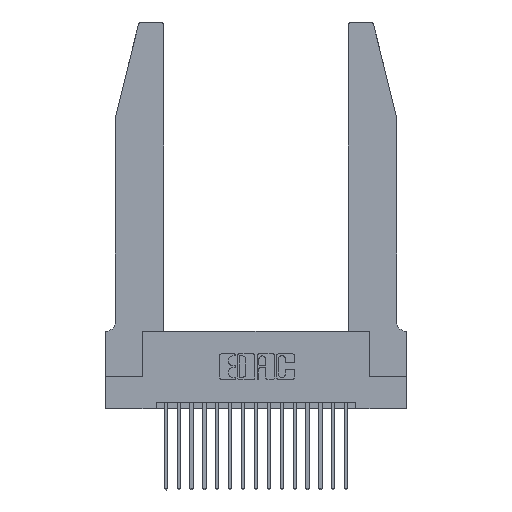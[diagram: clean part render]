
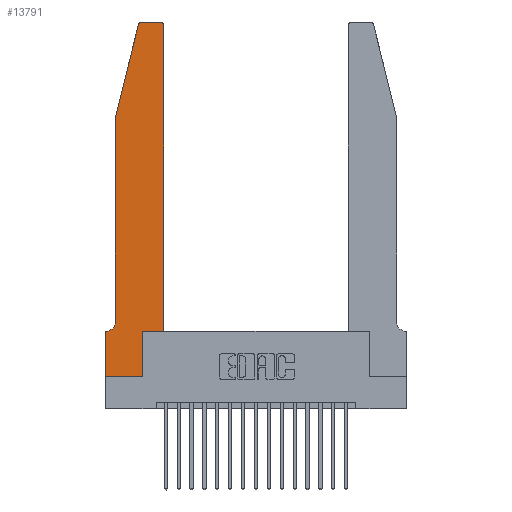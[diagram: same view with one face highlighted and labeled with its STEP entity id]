
A CAD part, top view. The second image highlights one B-rep face of the part: STEP entity #13791.
In plain terms, the highlighted planar face has unit normal (0, 0, 1).
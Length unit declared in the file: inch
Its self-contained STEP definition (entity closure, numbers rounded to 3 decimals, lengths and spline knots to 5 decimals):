
#321 = VECTOR ( 'NONE', #2564, 39.37008 ) ;
#482 = DIRECTION ( 'NONE',  ( 0., 0., 1. ) ) ;
#614 = DIRECTION ( 'NONE',  ( 1., 0., 0. ) ) ;
#712 = LINE ( 'NONE', #5059, #16830 ) ;
#840 = EDGE_CURVE ( 'NONE', #8991, #19075, #1540, .T. ) ;
#1194 = LINE ( 'NONE', #5356, #11461 ) ;
#1308 = DIRECTION ( 'NONE',  ( -0.239, -0.971, 0. ) ) ;
#1516 = VERTEX_POINT ( 'NONE', #19237 ) ;
#1540 = LINE ( 'NONE', #11918, #321 ) ;
#1639 = EDGE_CURVE ( 'NONE', #1516, #4636, #4676, .T. ) ;
#1781 = AXIS2_PLACEMENT_3D ( 'NONE', #9828, #482, #614 ) ;
#2176 = CIRCLE ( 'NONE', #12834, 0.03 ) ;
#2214 = ORIENTED_EDGE ( 'NONE', *, *, #1639, .T. ) ;
#2389 = VERTEX_POINT ( 'NONE', #17861 ) ;
#2411 = ORIENTED_EDGE ( 'NONE', *, *, #15832, .T. ) ;
#2564 = DIRECTION ( 'NONE',  ( 0., 1., 0. ) ) ;
#2669 = LINE ( 'NONE', #11225, #6383 ) ;
#3436 = VECTOR ( 'NONE', #15116, 39.37008 ) ;
#3654 = LINE ( 'NONE', #7555, #7358 ) ;
#4007 = CARTESIAN_POINT ( 'NONE',  ( 0.2865, 0., 0.37 ) ) ;
#4327 = PLANE ( 'NONE',  #1781 ) ;
#4636 = VERTEX_POINT ( 'NONE', #15361 ) ;
#4676 = LINE ( 'NONE', #11887, #3436 ) ;
#5059 = CARTESIAN_POINT ( 'NONE',  ( 0.4505, 0.35, 0.37 ) ) ;
#5154 = DIRECTION ( 'NONE',  ( -1., 0., 0. ) ) ;
#5286 = DIRECTION ( 'NONE',  ( 0., 1., 0. ) ) ;
#5349 = ORIENTED_EDGE ( 'NONE', *, *, #840, .T. ) ;
#5356 = CARTESIAN_POINT ( 'NONE',  ( 0.2865, 0.35, 0.37 ) ) ;
#5505 = ORIENTED_EDGE ( 'NONE', *, *, #15750, .T. ) ;
#5670 = EDGE_LOOP ( 'NONE', ( #7235, #18676, #13101, #5505, #6916, #6744, #2214, #2411, #11901, #12534, #5349, #15913 ) ) ;
#6383 = VECTOR ( 'NONE', #5154, 39.37008 ) ;
#6478 = VERTEX_POINT ( 'NONE', #4007 ) ;
#6493 = LINE ( 'NONE', #14521, #8422 ) ;
#6744 = ORIENTED_EDGE ( 'NONE', *, *, #15393, .T. ) ;
#6821 = DIRECTION ( 'NONE',  ( -1., 0., 0. ) ) ;
#6852 = VECTOR ( 'NONE', #12514, 39.37008 ) ;
#6901 = CIRCLE ( 'NONE', #7933, 0.03 ) ;
#6916 = ORIENTED_EDGE ( 'NONE', *, *, #7870, .T. ) ;
#7235 = ORIENTED_EDGE ( 'NONE', *, *, #7474, .T. ) ;
#7358 = VECTOR ( 'NONE', #1308, 39.37008 ) ;
#7474 = EDGE_CURVE ( 'NONE', #12507, #13814, #6493, .T. ) ;
#7505 = VERTEX_POINT ( 'NONE', #18657 ) ;
#7555 = CARTESIAN_POINT ( 'NONE',  ( 0.0755, 2., 0.37 ) ) ;
#7870 = EDGE_CURVE ( 'NONE', #2389, #10041, #16198, .T. ) ;
#7933 = AXIS2_PLACEMENT_3D ( 'NONE', #17990, #17774, #19406 ) ;
#8116 = DIRECTION ( 'NONE',  ( 1., 0., 0. ) ) ;
#8186 = DIRECTION ( 'NONE',  ( 0., 0., 1. ) ) ;
#8422 = VECTOR ( 'NONE', #6821, 39.37008 ) ;
#8977 = CARTESIAN_POINT ( 'NONE',  ( 0.0055, 0.42, 0.37 ) ) ;
#8991 = VERTEX_POINT ( 'NONE', #12371 ) ;
#9189 = CARTESIAN_POINT ( 'NONE',  ( 0.0755, 2., 0.37 ) ) ;
#9696 = CARTESIAN_POINT ( 'NONE',  ( 0.25487, 2.72718, 0.37 ) ) ;
#9828 = CARTESIAN_POINT ( 'NONE',  ( 0., 0.35, 0.37 ) ) ;
#10041 = VERTEX_POINT ( 'NONE', #16315 ) ;
#10943 = CARTESIAN_POINT ( 'NONE',  ( 0., 0., 0.37 ) ) ;
#11225 = CARTESIAN_POINT ( 'NONE',  ( 0.0755, 0.35, 0.37 ) ) ;
#11461 = VECTOR ( 'NONE', #5286, 39.37008 ) ;
#11567 = CARTESIAN_POINT ( 'NONE',  ( 0.4205, 2.75, 0.37 ) ) ;
#11744 = CARTESIAN_POINT ( 'NONE',  ( 0.284, 2.75, 0.37 ) ) ;
#11887 = CARTESIAN_POINT ( 'NONE',  ( 0., 0., 0.37 ) ) ;
#11901 = ORIENTED_EDGE ( 'NONE', *, *, #15420, .T. ) ;
#11918 = CARTESIAN_POINT ( 'NONE',  ( 0.4505, 0.35, 0.37 ) ) ;
#11966 = DIRECTION ( 'NONE',  ( -1., 0., 0. ) ) ;
#12099 = DIRECTION ( 'NONE',  ( 0., -1., 0. ) ) ;
#12371 = CARTESIAN_POINT ( 'NONE',  ( 0.4505, 0.35, 0.37 ) ) ;
#12507 = VERTEX_POINT ( 'NONE', #11567 ) ;
#12514 = DIRECTION ( 'NONE',  ( 1., 0., 0. ) ) ;
#12534 = ORIENTED_EDGE ( 'NONE', *, *, #17698, .T. ) ;
#12669 = VECTOR ( 'NONE', #12099, 39.37008 ) ;
#12834 = AXIS2_PLACEMENT_3D ( 'NONE', #19123, #8186, #8116 ) ;
#13101 = ORIENTED_EDGE ( 'NONE', *, *, #17579, .T. ) ;
#13640 = LINE ( 'NONE', #10943, #6852 ) ;
#13791 = ADVANCED_FACE ( 'NONE', ( #20083 ), #4327, .T. ) ;
#13814 = VERTEX_POINT ( 'NONE', #11744 ) ;
#14454 = CARTESIAN_POINT ( 'NONE',  ( 0.2865, 0.35, 0.37 ) ) ;
#14521 = CARTESIAN_POINT ( 'NONE',  ( 0.2605, 2.75, 0.37 ) ) ;
#15116 = DIRECTION ( 'NONE',  ( 0., -1., 0. ) ) ;
#15253 = EDGE_CURVE ( 'NONE', #13814, #16036, #2176, .T. ) ;
#15361 = CARTESIAN_POINT ( 'NONE',  ( 0., 0., 0.37 ) ) ;
#15393 = EDGE_CURVE ( 'NONE', #10041, #1516, #2669, .T. ) ;
#15407 = VERTEX_POINT ( 'NONE', #14454 ) ;
#15420 = EDGE_CURVE ( 'NONE', #6478, #15407, #1194, .T. ) ;
#15750 = EDGE_CURVE ( 'NONE', #7505, #2389, #16817, .T. ) ;
#15832 = EDGE_CURVE ( 'NONE', #4636, #6478, #13640, .T. ) ;
#15913 = ORIENTED_EDGE ( 'NONE', *, *, #16787, .T. ) ;
#16036 = VERTEX_POINT ( 'NONE', #9696 ) ;
#16125 = CARTESIAN_POINT ( 'NONE',  ( 0.4505, 2.72, 0.37 ) ) ;
#16198 = CIRCLE ( 'NONE', #16221, 0.07 ) ;
#16221 = AXIS2_PLACEMENT_3D ( 'NONE', #8977, #19589, #11966 ) ;
#16315 = CARTESIAN_POINT ( 'NONE',  ( 0.0055, 0.35, 0.37 ) ) ;
#16787 = EDGE_CURVE ( 'NONE', #19075, #12507, #6901, .T. ) ;
#16817 = LINE ( 'NONE', #9189, #12669 ) ;
#16830 = VECTOR ( 'NONE', #19102, 39.37008 ) ;
#17579 = EDGE_CURVE ( 'NONE', #16036, #7505, #3654, .T. ) ;
#17698 = EDGE_CURVE ( 'NONE', #15407, #8991, #712, .T. ) ;
#17774 = DIRECTION ( 'NONE',  ( 0., 0., 1. ) ) ;
#17861 = CARTESIAN_POINT ( 'NONE',  ( 0.0755, 0.42, 0.37 ) ) ;
#17990 = CARTESIAN_POINT ( 'NONE',  ( 0.4205, 2.72, 0.37 ) ) ;
#18657 = CARTESIAN_POINT ( 'NONE',  ( 0.0755, 2., 0.37 ) ) ;
#18676 = ORIENTED_EDGE ( 'NONE', *, *, #15253, .T. ) ;
#19075 = VERTEX_POINT ( 'NONE', #16125 ) ;
#19102 = DIRECTION ( 'NONE',  ( 1., 0., 0. ) ) ;
#19123 = CARTESIAN_POINT ( 'NONE',  ( 0.284, 2.72, 0.37 ) ) ;
#19237 = CARTESIAN_POINT ( 'NONE',  ( 0., 0.35, 0.37 ) ) ;
#19406 = DIRECTION ( 'NONE',  ( 1., 0., 0. ) ) ;
#19589 = DIRECTION ( 'NONE',  ( 0., 0., -1. ) ) ;
#20083 = FACE_OUTER_BOUND ( 'NONE', #5670, .T. ) ;
